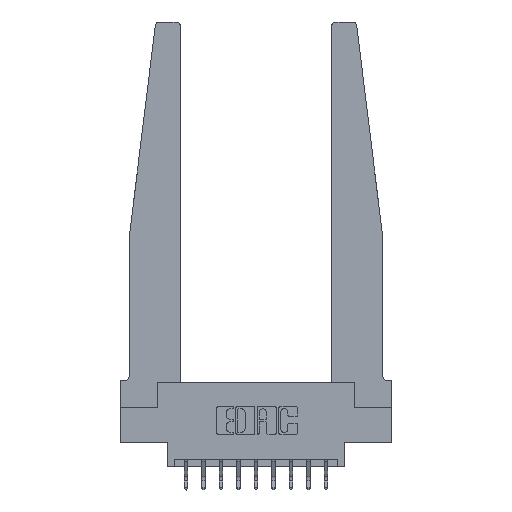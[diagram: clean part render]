
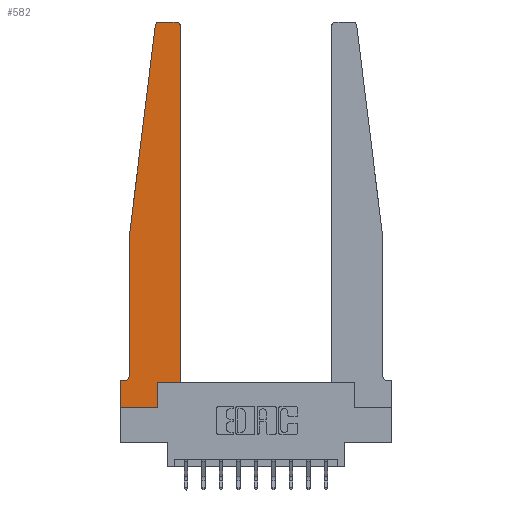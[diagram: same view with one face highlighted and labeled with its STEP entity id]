
A CAD part, top view. The second image highlights one B-rep face of the part: STEP entity #582.
In plain terms, the highlighted planar face has unit normal (0, 0, 1).
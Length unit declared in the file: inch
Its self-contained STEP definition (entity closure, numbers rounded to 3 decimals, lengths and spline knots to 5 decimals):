
#72 = DIRECTION ( 'NONE',  ( 0., 1., 0. ) ) ;
#73 = CARTESIAN_POINT ( 'NONE',  ( 0., 0., 0.37 ) ) ;
#375 = VERTEX_POINT ( 'NONE', #9352 ) ;
#449 = CARTESIAN_POINT ( 'NONE',  ( 0.425, 2.72, 0.37 ) ) ;
#532 = EDGE_CURVE ( 'NONE', #3370, #6709, #8913, .T. ) ;
#582 = ADVANCED_FACE ( 'NONE', ( #1781 ), #12835, .T. ) ;
#593 = CARTESIAN_POINT ( 'NONE',  ( 0.065, 0.2375, 0.37 ) ) ;
#752 = VECTOR ( 'NONE', #5652, 39.37008 ) ;
#887 = EDGE_CURVE ( 'NONE', #5722, #3370, #1591, .T. ) ;
#1117 = DIRECTION ( 'NONE',  ( 1., 0., 0. ) ) ;
#1366 = EDGE_CURVE ( 'NONE', #6709, #10970, #10989, .T. ) ;
#1403 = DIRECTION ( 'NONE',  ( 0., 0., -1. ) ) ;
#1533 = DIRECTION ( 'NONE',  ( 0., 0., 1. ) ) ;
#1569 = VERTEX_POINT ( 'NONE', #11295 ) ;
#1591 = CIRCLE ( 'NONE', #2840, 0.03 ) ;
#1781 = FACE_OUTER_BOUND ( 'NONE', #2548, .T. ) ;
#2003 = CARTESIAN_POINT ( 'NONE',  ( 0.25, 2.75, 0.37 ) ) ;
#2112 = DIRECTION ( 'NONE',  ( 1., 0., 0. ) ) ;
#2309 = EDGE_CURVE ( 'NONE', #7596, #375, #4932, .T. ) ;
#2369 = ORIENTED_EDGE ( 'NONE', *, *, #1366, .T. ) ;
#2548 = EDGE_LOOP ( 'NONE', ( #3634, #2369, #11048, #10969, #4994, #11403, #7955, #11768, #14438, #3388, #3767, #3644 ) ) ;
#2740 = VERTEX_POINT ( 'NONE', #593 ) ;
#2798 = VECTOR ( 'NONE', #72, 39.37008 ) ;
#2840 = AXIS2_PLACEMENT_3D ( 'NONE', #8712, #1533, #9909 ) ;
#2873 = EDGE_CURVE ( 'NONE', #10970, #3378, #13364, .T. ) ;
#3268 = CARTESIAN_POINT ( 'NONE',  ( 0., 0.1875, 0.37 ) ) ;
#3272 = VECTOR ( 'NONE', #13201, 39.37008 ) ;
#3370 = VERTEX_POINT ( 'NONE', #13793 ) ;
#3378 = VERTEX_POINT ( 'NONE', #14967 ) ;
#3388 = ORIENTED_EDGE ( 'NONE', *, *, #10160, .T. ) ;
#3486 = CIRCLE ( 'NONE', #15182, 0.05 ) ;
#3634 = ORIENTED_EDGE ( 'NONE', *, *, #532, .T. ) ;
#3644 = ORIENTED_EDGE ( 'NONE', *, *, #887, .T. ) ;
#3767 = ORIENTED_EDGE ( 'NONE', *, *, #4632, .T. ) ;
#3942 = CARTESIAN_POINT ( 'NONE',  ( 0., 0., 0.37 ) ) ;
#4632 = EDGE_CURVE ( 'NONE', #1569, #5722, #13115, .T. ) ;
#4824 = VECTOR ( 'NONE', #1117, 39.37008 ) ;
#4932 = LINE ( 'NONE', #14042, #8138 ) ;
#4976 = EDGE_CURVE ( 'NONE', #5671, #13202, #12163, .T. ) ;
#4994 = ORIENTED_EDGE ( 'NONE', *, *, #14110, .T. ) ;
#5650 = CARTESIAN_POINT ( 'NONE',  ( 0.065, 1.25, 0.37 ) ) ;
#5652 = DIRECTION ( 'NONE',  ( 0., -1., 0. ) ) ;
#5671 = VERTEX_POINT ( 'NONE', #3942 ) ;
#5714 = VECTOR ( 'NONE', #10399, 39.37008 ) ;
#5722 = VERTEX_POINT ( 'NONE', #449 ) ;
#6120 = DIRECTION ( 'NONE',  ( 0., 0., 1. ) ) ;
#6709 = VERTEX_POINT ( 'NONE', #14416 ) ;
#6880 = DIRECTION ( 'NONE',  ( -1., 0., 0. ) ) ;
#7094 = CARTESIAN_POINT ( 'NONE',  ( 0.425, 0.18, 0.37 ) ) ;
#7365 = VECTOR ( 'NONE', #15202, 39.37008 ) ;
#7494 = LINE ( 'NONE', #9224, #752 ) ;
#7580 = DIRECTION ( 'NONE',  ( 1., 0., 0. ) ) ;
#7587 = LINE ( 'NONE', #73, #3272 ) ;
#7596 = VERTEX_POINT ( 'NONE', #14853 ) ;
#7955 = ORIENTED_EDGE ( 'NONE', *, *, #12260, .T. ) ;
#8138 = VECTOR ( 'NONE', #6880, 39.37008 ) ;
#8246 = VECTOR ( 'NONE', #7580, 39.37008 ) ;
#8428 = CARTESIAN_POINT ( 'NONE',  ( 0.2605, 0.18, 0.37 ) ) ;
#8436 = CARTESIAN_POINT ( 'NONE',  ( 0.2605, 0.18, 0.37 ) ) ;
#8592 = CARTESIAN_POINT ( 'NONE',  ( 0.015, 0.2375, 0.37 ) ) ;
#8712 = CARTESIAN_POINT ( 'NONE',  ( 0.395, 2.72, 0.37 ) ) ;
#8913 = LINE ( 'NONE', #2003, #5714 ) ;
#8954 = EDGE_CURVE ( 'NONE', #3378, #2740, #7494, .T. ) ;
#9104 = EDGE_CURVE ( 'NONE', #13202, #10865, #11599, .T. ) ;
#9224 = CARTESIAN_POINT ( 'NONE',  ( 0.065, 1.25, 0.37 ) ) ;
#9295 = DIRECTION ( 'NONE',  ( 0., 0., 1. ) ) ;
#9352 = CARTESIAN_POINT ( 'NONE',  ( 0., 0.1875, 0.37 ) ) ;
#9567 = AXIS2_PLACEMENT_3D ( 'NONE', #3268, #9295, #2112 ) ;
#9787 = DIRECTION ( 'NONE',  ( -1., 0., 0. ) ) ;
#9909 = DIRECTION ( 'NONE',  ( 1., 0., 0. ) ) ;
#10160 = EDGE_CURVE ( 'NONE', #10865, #1569, #14361, .T. ) ;
#10399 = DIRECTION ( 'NONE',  ( -1., 0., 0. ) ) ;
#10865 = VERTEX_POINT ( 'NONE', #8428 ) ;
#10969 = ORIENTED_EDGE ( 'NONE', *, *, #8954, .T. ) ;
#10970 = VERTEX_POINT ( 'NONE', #11000 ) ;
#10989 = CIRCLE ( 'NONE', #14565, 0.03 ) ;
#11000 = CARTESIAN_POINT ( 'NONE',  ( 0.24675, 2.72367, 0.37 ) ) ;
#11048 = ORIENTED_EDGE ( 'NONE', *, *, #2873, .T. ) ;
#11295 = CARTESIAN_POINT ( 'NONE',  ( 0.425, 0.18, 0.37 ) ) ;
#11403 = ORIENTED_EDGE ( 'NONE', *, *, #2309, .T. ) ;
#11512 = CARTESIAN_POINT ( 'NONE',  ( 0.425, 0.18, 0.37 ) ) ;
#11599 = LINE ( 'NONE', #8436, #2798 ) ;
#11768 = ORIENTED_EDGE ( 'NONE', *, *, #4976, .T. ) ;
#12163 = LINE ( 'NONE', #14720, #8246 ) ;
#12260 = EDGE_CURVE ( 'NONE', #375, #5671, #7587, .T. ) ;
#12358 = VECTOR ( 'NONE', #12700, 39.37008 ) ;
#12700 = DIRECTION ( 'NONE',  ( 0., 1., 0. ) ) ;
#12835 = PLANE ( 'NONE',  #9567 ) ;
#13115 = LINE ( 'NONE', #11512, #12358 ) ;
#13201 = DIRECTION ( 'NONE',  ( 0., -1., 0. ) ) ;
#13202 = VERTEX_POINT ( 'NONE', #15224 ) ;
#13294 = CARTESIAN_POINT ( 'NONE',  ( 0.27653, 2.72, 0.37 ) ) ;
#13364 = LINE ( 'NONE', #5650, #7365 ) ;
#13793 = CARTESIAN_POINT ( 'NONE',  ( 0.395, 2.75, 0.37 ) ) ;
#14042 = CARTESIAN_POINT ( 'NONE',  ( 0.065, 0.1875, 0.37 ) ) ;
#14110 = EDGE_CURVE ( 'NONE', #2740, #7596, #3486, .T. ) ;
#14361 = LINE ( 'NONE', #7094, #4824 ) ;
#14416 = CARTESIAN_POINT ( 'NONE',  ( 0.27653, 2.75, 0.37 ) ) ;
#14438 = ORIENTED_EDGE ( 'NONE', *, *, #9104, .T. ) ;
#14478 = DIRECTION ( 'NONE',  ( 1., 0., 0. ) ) ;
#14565 = AXIS2_PLACEMENT_3D ( 'NONE', #13294, #6120, #14478 ) ;
#14720 = CARTESIAN_POINT ( 'NONE',  ( 0., 0., 0.37 ) ) ;
#14853 = CARTESIAN_POINT ( 'NONE',  ( 0.015, 0.1875, 0.37 ) ) ;
#14967 = CARTESIAN_POINT ( 'NONE',  ( 0.065, 1.25, 0.37 ) ) ;
#15182 = AXIS2_PLACEMENT_3D ( 'NONE', #8592, #1403, #9787 ) ;
#15202 = DIRECTION ( 'NONE',  ( -0.122, -0.992, 0. ) ) ;
#15224 = CARTESIAN_POINT ( 'NONE',  ( 0.2605, 0., 0.37 ) ) ;
